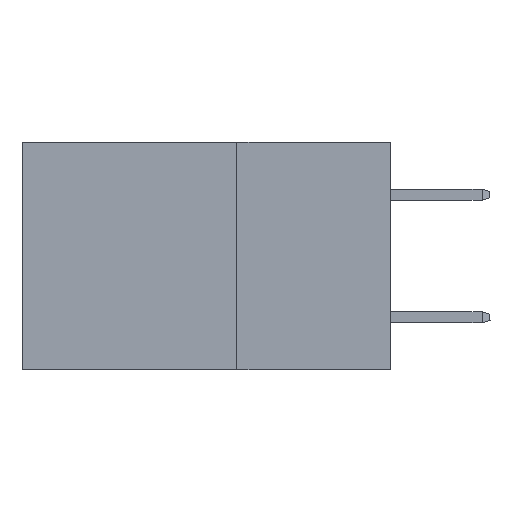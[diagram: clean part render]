
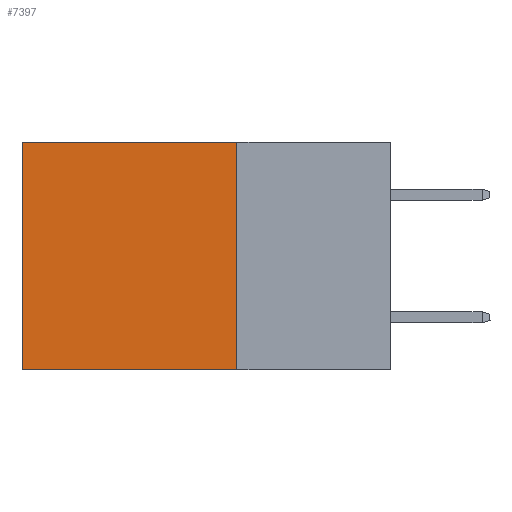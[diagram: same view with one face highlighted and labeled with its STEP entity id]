
A CAD part, left-side view. The second image highlights one B-rep face of the part: STEP entity #7397.
In plain terms, the highlighted planar face has unit normal (-1, 0, 0).
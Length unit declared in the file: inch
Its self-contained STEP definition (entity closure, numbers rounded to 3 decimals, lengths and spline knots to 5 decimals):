
#383 = VECTOR ( 'NONE', #3316, 39.37008 ) ;
#589 = CARTESIAN_POINT ( 'NONE',  ( 0.2875, 0.25, 0. ) ) ;
#664 = FACE_OUTER_BOUND ( 'NONE', #5515, .T. ) ;
#793 = VERTEX_POINT ( 'NONE', #9333 ) ;
#1099 = CARTESIAN_POINT ( 'NONE',  ( 0.2875, 0.25, -0.37 ) ) ;
#1345 = ORIENTED_EDGE ( 'NONE', *, *, #5572, .T. ) ;
#1586 = CARTESIAN_POINT ( 'NONE',  ( 0.2875, 0.25, 0. ) ) ;
#1651 = LINE ( 'NONE', #9426, #8074 ) ;
#2070 = DIRECTION ( 'NONE',  ( 0., 1., 0. ) ) ;
#2218 = PLANE ( 'NONE',  #5026 ) ;
#3316 = DIRECTION ( 'NONE',  ( 0., 0., -1. ) ) ;
#3915 = CARTESIAN_POINT ( 'NONE',  ( 0.2875, 0.25, 0. ) ) ;
#4238 = VERTEX_POINT ( 'NONE', #7149 ) ;
#4257 = EDGE_CURVE ( 'NONE', #793, #8556, #6754, .T. ) ;
#4505 = VECTOR ( 'NONE', #2070, 39.37008 ) ;
#5026 = AXIS2_PLACEMENT_3D ( 'NONE', #3915, #11029, #5616 ) ;
#5121 = LINE ( 'NONE', #9540, #10248 ) ;
#5372 = ORIENTED_EDGE ( 'NONE', *, *, #5509, .T. ) ;
#5509 = EDGE_CURVE ( 'NONE', #6865, #4238, #1651, .T. ) ;
#5515 = EDGE_LOOP ( 'NONE', ( #1345, #10257, #5646, #5372 ) ) ;
#5568 = EDGE_CURVE ( 'NONE', #6865, #793, #10530, .T. ) ;
#5572 = EDGE_CURVE ( 'NONE', #4238, #8556, #5121, .T. ) ;
#5616 = DIRECTION ( 'NONE',  ( 0., 0., -1. ) ) ;
#5646 = ORIENTED_EDGE ( 'NONE', *, *, #5568, .F. ) ;
#5772 = DIRECTION ( 'NONE',  ( 0., 1., 0. ) ) ;
#6442 = CARTESIAN_POINT ( 'NONE',  ( 0.2875, 0.6, -0.37 ) ) ;
#6754 = LINE ( 'NONE', #1099, #4505 ) ;
#6865 = VERTEX_POINT ( 'NONE', #589 ) ;
#7149 = CARTESIAN_POINT ( 'NONE',  ( 0.2875, 0.6, 0. ) ) ;
#7397 = ADVANCED_FACE ( 'NONE', ( #664 ), #2218, .F. ) ;
#8074 = VECTOR ( 'NONE', #5772, 39.37008 ) ;
#8556 = VERTEX_POINT ( 'NONE', #6442 ) ;
#9333 = CARTESIAN_POINT ( 'NONE',  ( 0.2875, 0.25, -0.37 ) ) ;
#9426 = CARTESIAN_POINT ( 'NONE',  ( 0.2875, 0.25, 0. ) ) ;
#9540 = CARTESIAN_POINT ( 'NONE',  ( 0.2875, 0.6, 0. ) ) ;
#10248 = VECTOR ( 'NONE', #10477, 39.37008 ) ;
#10257 = ORIENTED_EDGE ( 'NONE', *, *, #4257, .F. ) ;
#10477 = DIRECTION ( 'NONE',  ( 0., 0., -1. ) ) ;
#10530 = LINE ( 'NONE', #1586, #383 ) ;
#11029 = DIRECTION ( 'NONE',  ( 1., 0., 0. ) ) ;
